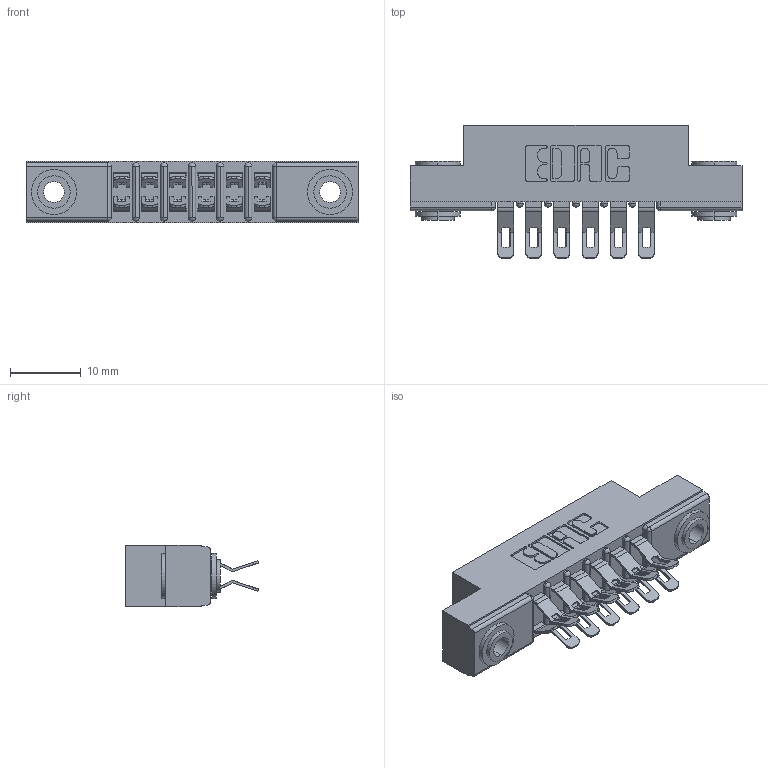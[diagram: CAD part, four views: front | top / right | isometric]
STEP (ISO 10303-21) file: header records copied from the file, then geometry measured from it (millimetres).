
FILE_DESCRIPTION (( 'STEP AP203' ), '1' );
FILE_NAME ('357-012-555-203.STEP', '2019-09-17T18:04:02', ( '' ), ( '' ), 'SwSTEP 2.0', 'SolidWorks 2016', '' );
FILE_SCHEMA (( 'CONFIG_CONTROL_DESIGN' ));
Length unit declared in the file: inch
Products named in the file (4): 345-250-002_345-250-002-102; 307-290-001_555; 357-012-555-203; 307 Part_.156 Dia Mounting Holes
Assembly tree (15 placements, depth 2):
  357-012-555-203
    307 Part_.156 Dia Mounting Holes
    307-290-001_555  x12
    345-250-002_345-250-002-102  x2
Bounding box: 46.79 x 18.75 x 8.71 mm (x, y, z)
Volume: 3099.2 mm3; surface area: 5084.3 mm2
Topology: 15 solids, 15 shells, 909 faces, 2607 edges, 1698 vertices
Faces by surface type: plane 502, cylinder 385, sphere 14, cone 8
Entity records: 11376 total; most frequent: CARTESIAN_POINT 1859, DIRECTION 1858, ORIENTED_EDGE 1832, EDGE_CURVE 916, LINE 668, VECTOR 668, VERTEX_POINT 596, AXIS2_PLACEMENT_3D 595
